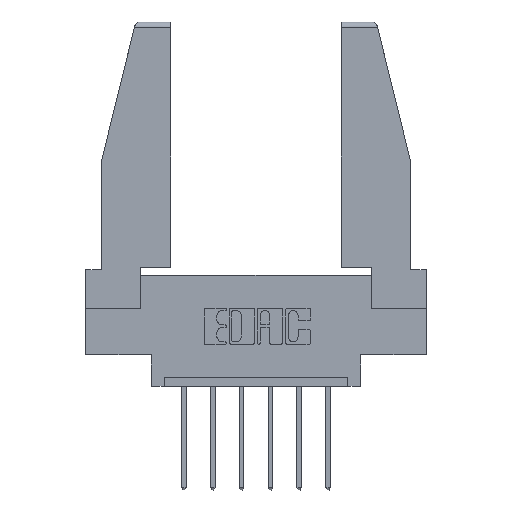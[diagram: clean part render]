
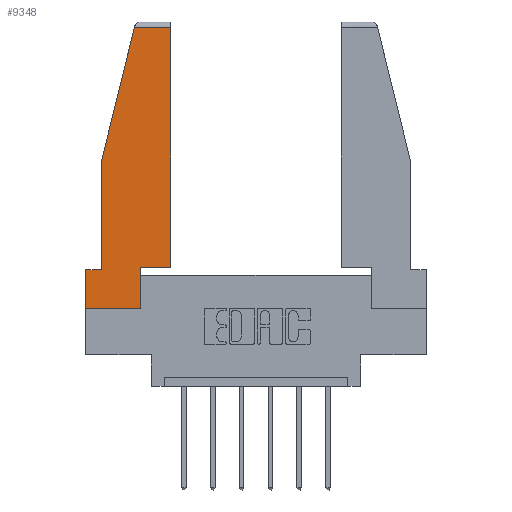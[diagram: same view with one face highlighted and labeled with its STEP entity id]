
A CAD part, top view. The second image highlights one B-rep face of the part: STEP entity #9348.
In plain terms, the highlighted planar face has unit normal (0, 0, 1).
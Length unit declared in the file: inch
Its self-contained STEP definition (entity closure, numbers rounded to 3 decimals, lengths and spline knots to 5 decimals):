
#109 = LINE ( 'NONE', #474, #400 ) ;
#223 = CARTESIAN_POINT ( 'NONE',  ( 0.086, 0.21, 0. ) ) ;
#233 = AXIS2_PLACEMENT_3D ( 'NONE', #8926, #4456, #6195 ) ;
#400 = VECTOR ( 'NONE', #7727, 39.37008 ) ;
#474 = CARTESIAN_POINT ( 'NONE',  ( 0., 0.21, 0. ) ) ;
#639 = ORIENTED_EDGE ( 'NONE', *, *, #11514, .T. ) ;
#746 = VECTOR ( 'NONE', #9578, 39.37008 ) ;
#898 = VECTOR ( 'NONE', #6968, 39.37008 ) ;
#1298 = VECTOR ( 'NONE', #9811, 39.37008 ) ;
#1997 = VERTEX_POINT ( 'NONE', #4481 ) ;
#2175 = LINE ( 'NONE', #11014, #7513 ) ;
#2729 = VERTEX_POINT ( 'NONE', #4114 ) ;
#2736 = VECTOR ( 'NONE', #8879, 39.37008 ) ;
#3151 = VERTEX_POINT ( 'NONE', #3517 ) ;
#3183 = EDGE_CURVE ( 'NONE', #10679, #8928, #3448, .T. ) ;
#3416 = CARTESIAN_POINT ( 'NONE',  ( 0.271, 1.55, 0. ) ) ;
#3448 = LINE ( 'NONE', #11579, #898 ) ;
#3515 = VERTEX_POINT ( 'NONE', #9324 ) ;
#3517 = CARTESIAN_POINT ( 'NONE',  ( 0., 0., 0. ) ) ;
#4040 = EDGE_CURVE ( 'NONE', #8928, #6793, #6651, .T. ) ;
#4114 = CARTESIAN_POINT ( 'NONE',  ( 0.461, 0.223, 0. ) ) ;
#4175 = CARTESIAN_POINT ( 'NONE',  ( 0., 0., 0. ) ) ;
#4456 = DIRECTION ( 'NONE',  ( 0., 0., 1. ) ) ;
#4481 = CARTESIAN_POINT ( 'NONE',  ( 0.2636, 1.52, 0. ) ) ;
#4543 = CARTESIAN_POINT ( 'NONE',  ( 0.086, 0.8, 0. ) ) ;
#4700 = LINE ( 'NONE', #8992, #2736 ) ;
#5033 = CARTESIAN_POINT ( 'NONE',  ( 0.297, 0.223, 0. ) ) ;
#5112 = ORIENTED_EDGE ( 'NONE', *, *, #5416, .T. ) ;
#5416 = EDGE_CURVE ( 'NONE', #8203, #2729, #6218, .T. ) ;
#5827 = FACE_OUTER_BOUND ( 'NONE', #8081, .T. ) ;
#6057 = LINE ( 'NONE', #7641, #9876 ) ;
#6160 = EDGE_CURVE ( 'NONE', #3515, #8203, #6057, .T. ) ;
#6195 = DIRECTION ( 'NONE',  ( 1., 0., 0. ) ) ;
#6218 = LINE ( 'NONE', #9289, #10756 ) ;
#6400 = ORIENTED_EDGE ( 'NONE', *, *, #3183, .T. ) ;
#6477 = EDGE_CURVE ( 'NONE', #6793, #3151, #109, .T. ) ;
#6651 = LINE ( 'NONE', #9534, #746 ) ;
#6793 = VERTEX_POINT ( 'NONE', #7489 ) ;
#6847 = CARTESIAN_POINT ( 'NONE',  ( 0.461, 1.52, 0. ) ) ;
#6968 = DIRECTION ( 'NONE',  ( 0., -1., 0. ) ) ;
#7321 = LINE ( 'NONE', #4175, #9164 ) ;
#7432 = ORIENTED_EDGE ( 'NONE', *, *, #4040, .T. ) ;
#7489 = CARTESIAN_POINT ( 'NONE',  ( 0., 0.21, 0. ) ) ;
#7513 = VECTOR ( 'NONE', #11595, 39.37008 ) ;
#7641 = CARTESIAN_POINT ( 'NONE',  ( 0.297, 0., 0. ) ) ;
#7727 = DIRECTION ( 'NONE',  ( 0., -1., 0. ) ) ;
#7738 = ORIENTED_EDGE ( 'NONE', *, *, #6160, .T. ) ;
#8021 = PLANE ( 'NONE',  #233 ) ;
#8081 = EDGE_LOOP ( 'NONE', ( #9142, #9632, #9460, #6400, #7432, #10789, #639, #7738, #5112 ) ) ;
#8203 = VERTEX_POINT ( 'NONE', #5033 ) ;
#8364 = VERTEX_POINT ( 'NONE', #6847 ) ;
#8434 = DIRECTION ( 'NONE',  ( 1., 0., 0. ) ) ;
#8460 = EDGE_CURVE ( 'NONE', #8364, #1997, #4700, .T. ) ;
#8879 = DIRECTION ( 'NONE',  ( -1., 0., 0. ) ) ;
#8904 = EDGE_CURVE ( 'NONE', #2729, #8364, #2175, .T. ) ;
#8926 = CARTESIAN_POINT ( 'NONE',  ( 0., 0., 0. ) ) ;
#8928 = VERTEX_POINT ( 'NONE', #223 ) ;
#8992 = CARTESIAN_POINT ( 'NONE',  ( 0., 1.52, 0. ) ) ;
#9142 = ORIENTED_EDGE ( 'NONE', *, *, #8904, .T. ) ;
#9164 = VECTOR ( 'NONE', #10429, 39.37008 ) ;
#9187 = LINE ( 'NONE', #3416, #1298 ) ;
#9289 = CARTESIAN_POINT ( 'NONE',  ( 0.297, 0.223, 0. ) ) ;
#9324 = CARTESIAN_POINT ( 'NONE',  ( 0.297, 0., 0. ) ) ;
#9348 = ADVANCED_FACE ( 'NONE', ( #5827 ), #8021, .T. ) ;
#9460 = ORIENTED_EDGE ( 'NONE', *, *, #10593, .T. ) ;
#9534 = CARTESIAN_POINT ( 'NONE',  ( 0., 0.21, 0. ) ) ;
#9578 = DIRECTION ( 'NONE',  ( -1., 0., 0. ) ) ;
#9632 = ORIENTED_EDGE ( 'NONE', *, *, #8460, .T. ) ;
#9811 = DIRECTION ( 'NONE',  ( -0.239, -0.971, 0. ) ) ;
#9876 = VECTOR ( 'NONE', #11369, 39.37008 ) ;
#10429 = DIRECTION ( 'NONE',  ( 1., 0., 0. ) ) ;
#10593 = EDGE_CURVE ( 'NONE', #1997, #10679, #9187, .T. ) ;
#10679 = VERTEX_POINT ( 'NONE', #4543 ) ;
#10756 = VECTOR ( 'NONE', #8434, 39.37008 ) ;
#10789 = ORIENTED_EDGE ( 'NONE', *, *, #6477, .T. ) ;
#11014 = CARTESIAN_POINT ( 'NONE',  ( 0.461, 0.223, 0. ) ) ;
#11369 = DIRECTION ( 'NONE',  ( 0., 1., 0. ) ) ;
#11514 = EDGE_CURVE ( 'NONE', #3151, #3515, #7321, .T. ) ;
#11579 = CARTESIAN_POINT ( 'NONE',  ( 0.086, 0.8, 0. ) ) ;
#11595 = DIRECTION ( 'NONE',  ( 0., 1., 0. ) ) ;
